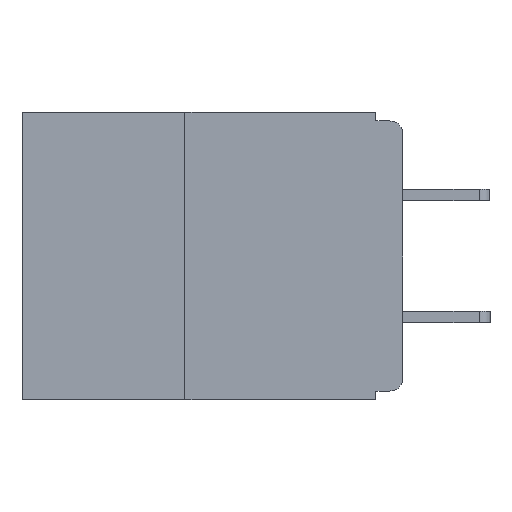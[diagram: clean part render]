
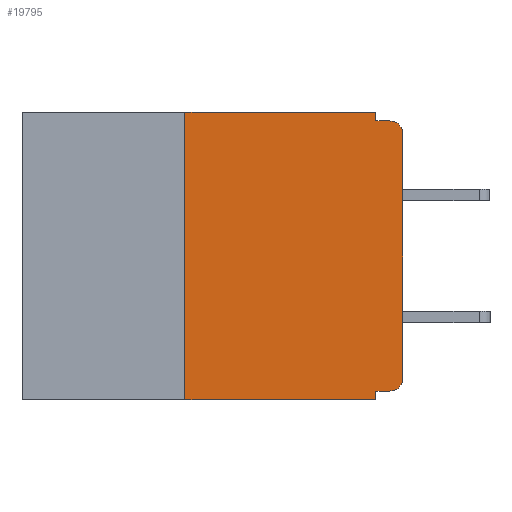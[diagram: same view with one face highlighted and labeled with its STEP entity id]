
A CAD part, left-side view. The second image highlights one B-rep face of the part: STEP entity #19795.
In plain terms, the highlighted planar face has unit normal (-1, 0, 0).
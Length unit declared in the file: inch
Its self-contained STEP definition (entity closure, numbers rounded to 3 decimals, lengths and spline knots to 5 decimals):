
#18 = CARTESIAN_POINT ( 'NONE',  ( 0., 0.437, -0.33 ) ) ;
#268 = CARTESIAN_POINT ( 'NONE',  ( 0., 0.437, 0. ) ) ;
#802 = CARTESIAN_POINT ( 'NONE',  ( 0., 0., -0.305 ) ) ;
#1019 = EDGE_CURVE ( 'NONE', #21254, #20985, #14815, .T. ) ;
#1746 = VERTEX_POINT ( 'NONE', #1936 ) ;
#1764 = CARTESIAN_POINT ( 'NONE',  ( 0., 0.031, -0.33 ) ) ;
#1772 = EDGE_CURVE ( 'NONE', #17010, #2834, #23890, .T. ) ;
#1936 = CARTESIAN_POINT ( 'NONE',  ( 0., 0.031, -0.32 ) ) ;
#2248 = DIRECTION ( 'NONE',  ( 0., -1., 0. ) ) ;
#2411 = DIRECTION ( 'NONE',  ( -1., 0., 0. ) ) ;
#2528 = CARTESIAN_POINT ( 'NONE',  ( 0., 0.437, 0. ) ) ;
#2666 = CARTESIAN_POINT ( 'NONE',  ( 0., 0.015, -0.32 ) ) ;
#2834 = VERTEX_POINT ( 'NONE', #802 ) ;
#3004 = CARTESIAN_POINT ( 'NONE',  ( 0., 0.25, -0.33 ) ) ;
#3191 = VERTEX_POINT ( 'NONE', #13588 ) ;
#3307 = LINE ( 'NONE', #1764, #18545 ) ;
#3425 = CARTESIAN_POINT ( 'NONE',  ( 0., 0., 0. ) ) ;
#3495 = CIRCLE ( 'NONE', #25004, 0.015 ) ;
#3767 = DIRECTION ( 'NONE',  ( 0., 0., -1. ) ) ;
#3793 = VECTOR ( 'NONE', #8375, 39.37008 ) ;
#3802 = DIRECTION ( 'NONE',  ( -1., 0., 0. ) ) ;
#3806 = VERTEX_POINT ( 'NONE', #8050 ) ;
#3832 = CARTESIAN_POINT ( 'NONE',  ( 0., 0.015, -0.025 ) ) ;
#4340 = CARTESIAN_POINT ( 'NONE',  ( 0., 0.031, 0. ) ) ;
#4547 = DIRECTION ( 'NONE',  ( 1., 0., 0. ) ) ;
#4600 = VERTEX_POINT ( 'NONE', #20360 ) ;
#4730 = DIRECTION ( 'NONE',  ( 0., 0., 1. ) ) ;
#6248 = VERTEX_POINT ( 'NONE', #25091 ) ;
#6752 = AXIS2_PLACEMENT_3D ( 'NONE', #20882, #2411, #22223 ) ;
#6916 = EDGE_CURVE ( 'NONE', #2834, #3191, #23766, .T. ) ;
#7525 = LINE ( 'NONE', #18, #23719 ) ;
#8050 = CARTESIAN_POINT ( 'NONE',  ( 0., 0.25, 0. ) ) ;
#8375 = DIRECTION ( 'NONE',  ( 0., 0., -1. ) ) ;
#8861 = EDGE_CURVE ( 'NONE', #3191, #6248, #3495, .T. ) ;
#10212 = AXIS2_PLACEMENT_3D ( 'NONE', #268, #4547, #18988 ) ;
#10644 = LINE ( 'NONE', #3004, #20841 ) ;
#10998 = EDGE_CURVE ( 'NONE', #3806, #21254, #22584, .T. ) ;
#11183 = VECTOR ( 'NONE', #2248, 39.37008 ) ;
#11238 = ORIENTED_EDGE ( 'NONE', *, *, #1772, .T. ) ;
#11408 = LINE ( 'NONE', #17827, #26138 ) ;
#12421 = VECTOR ( 'NONE', #4730, 39.37008 ) ;
#12435 = VERTEX_POINT ( 'NONE', #25274 ) ;
#12575 = DIRECTION ( 'NONE',  ( 0., -1., 0. ) ) ;
#12668 = CARTESIAN_POINT ( 'NONE',  ( 0., 0.031, -0.01 ) ) ;
#12955 = EDGE_CURVE ( 'NONE', #17010, #1746, #11408, .T. ) ;
#12987 = LINE ( 'NONE', #19662, #17836 ) ;
#13588 = CARTESIAN_POINT ( 'NONE',  ( 0., 0., -0.025 ) ) ;
#14028 = ORIENTED_EDGE ( 'NONE', *, *, #22475, .F. ) ;
#14248 = DIRECTION ( 'NONE',  ( 0., 0., -1. ) ) ;
#14346 = EDGE_LOOP ( 'NONE', ( #19191, #23060, #14028, #16927, #23795, #17796, #18102, #25231, #20431, #11238 ) ) ;
#14815 = LINE ( 'NONE', #21250, #3793 ) ;
#15479 = DIRECTION ( 'NONE',  ( 0., -1., 0. ) ) ;
#16905 = PLANE ( 'NONE',  #10212 ) ;
#16927 = ORIENTED_EDGE ( 'NONE', *, *, #1019, .F. ) ;
#17010 = VERTEX_POINT ( 'NONE', #2666 ) ;
#17796 = ORIENTED_EDGE ( 'NONE', *, *, #24919, .F. ) ;
#17827 = CARTESIAN_POINT ( 'NONE',  ( 0., 0., -0.32 ) ) ;
#17836 = VECTOR ( 'NONE', #15479, 39.37008 ) ;
#17853 = DIRECTION ( 'NONE',  ( 0., 1., 0. ) ) ;
#18102 = ORIENTED_EDGE ( 'NONE', *, *, #20974, .T. ) ;
#18545 = VECTOR ( 'NONE', #14248, 39.37008 ) ;
#18988 = DIRECTION ( 'NONE',  ( 0., 0., -1. ) ) ;
#19191 = ORIENTED_EDGE ( 'NONE', *, *, #6916, .T. ) ;
#19542 = DIRECTION ( 'NONE',  ( 0., 0., 1. ) ) ;
#19616 = EDGE_CURVE ( 'NONE', #1746, #12435, #3307, .T. ) ;
#19662 = CARTESIAN_POINT ( 'NONE',  ( 0., 0., -0.01 ) ) ;
#19795 = ADVANCED_FACE ( 'NONE', ( #24722 ), #16905, .F. ) ;
#20360 = CARTESIAN_POINT ( 'NONE',  ( 0., 0.25, -0.33 ) ) ;
#20431 = ORIENTED_EDGE ( 'NONE', *, *, #12955, .F. ) ;
#20841 = VECTOR ( 'NONE', #19542, 39.37008 ) ;
#20882 = CARTESIAN_POINT ( 'NONE',  ( 0., 0.015, -0.305 ) ) ;
#20974 = EDGE_CURVE ( 'NONE', #4600, #12435, #7525, .T. ) ;
#20985 = VERTEX_POINT ( 'NONE', #12668 ) ;
#21250 = CARTESIAN_POINT ( 'NONE',  ( 0., 0.031, 0. ) ) ;
#21254 = VERTEX_POINT ( 'NONE', #4340 ) ;
#22223 = DIRECTION ( 'NONE',  ( 0., 0., -1. ) ) ;
#22475 = EDGE_CURVE ( 'NONE', #20985, #6248, #12987, .T. ) ;
#22584 = LINE ( 'NONE', #2528, #11183 ) ;
#23060 = ORIENTED_EDGE ( 'NONE', *, *, #8861, .T. ) ;
#23719 = VECTOR ( 'NONE', #12575, 39.37008 ) ;
#23766 = LINE ( 'NONE', #3425, #12421 ) ;
#23795 = ORIENTED_EDGE ( 'NONE', *, *, #10998, .F. ) ;
#23890 = CIRCLE ( 'NONE', #6752, 0.015 ) ;
#24722 = FACE_OUTER_BOUND ( 'NONE', #14346, .T. ) ;
#24919 = EDGE_CURVE ( 'NONE', #4600, #3806, #10644, .T. ) ;
#25004 = AXIS2_PLACEMENT_3D ( 'NONE', #3832, #3802, #3767 ) ;
#25091 = CARTESIAN_POINT ( 'NONE',  ( 0., 0.015, -0.01 ) ) ;
#25231 = ORIENTED_EDGE ( 'NONE', *, *, #19616, .F. ) ;
#25274 = CARTESIAN_POINT ( 'NONE',  ( 0., 0.031, -0.33 ) ) ;
#26138 = VECTOR ( 'NONE', #17853, 39.37008 ) ;
